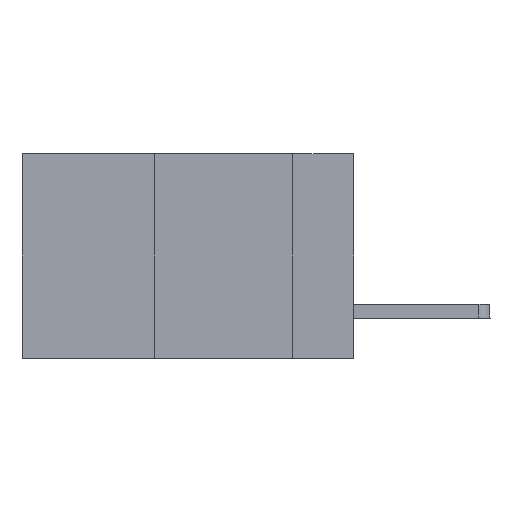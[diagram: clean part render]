
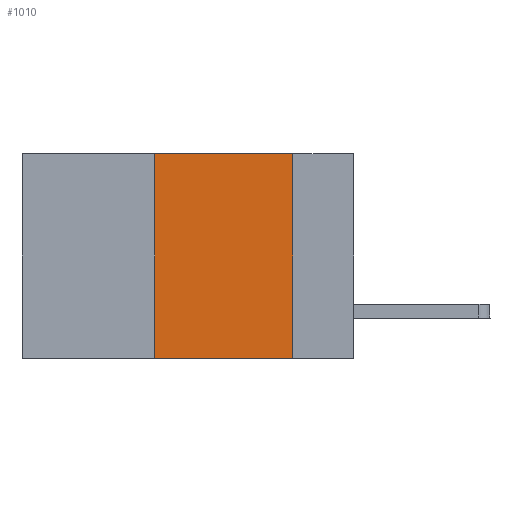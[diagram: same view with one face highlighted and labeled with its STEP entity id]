
A CAD part, left-side view. The second image highlights one B-rep face of the part: STEP entity #1010.
In plain terms, the highlighted planar face has unit normal (-1, 0, 0).
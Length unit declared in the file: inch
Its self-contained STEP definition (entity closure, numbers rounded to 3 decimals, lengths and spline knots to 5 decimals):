
#25 = VERTEX_POINT ( 'NONE', #12818 ) ;
#336 = EDGE_LOOP ( 'NONE', ( #13020, #1148, #7631, #9449 ) ) ;
#522 = CARTESIAN_POINT ( 'NONE',  ( 0., 0.11, 0. ) ) ;
#782 = CARTESIAN_POINT ( 'NONE',  ( 0., 0.11, -0.37 ) ) ;
#1010 = ADVANCED_FACE ( 'NONE', ( #8247 ), #4145, .F. ) ;
#1148 = ORIENTED_EDGE ( 'NONE', *, *, #11933, .F. ) ;
#1301 = VERTEX_POINT ( 'NONE', #7869 ) ;
#3230 = AXIS2_PLACEMENT_3D ( 'NONE', #7863, #12127, #12901 ) ;
#4145 = PLANE ( 'NONE',  #3230 ) ;
#4579 = DIRECTION ( 'NONE',  ( 0., -1., 0. ) ) ;
#4854 = VERTEX_POINT ( 'NONE', #522 ) ;
#6179 = CARTESIAN_POINT ( 'NONE',  ( 0., 0.36, 0. ) ) ;
#6302 = VECTOR ( 'NONE', #11400, 39.37008 ) ;
#6614 = VECTOR ( 'NONE', #4579, 39.37008 ) ;
#6627 = LINE ( 'NONE', #6179, #6302 ) ;
#7347 = DIRECTION ( 'NONE',  ( 0., -1., 0. ) ) ;
#7631 = ORIENTED_EDGE ( 'NONE', *, *, #13656, .F. ) ;
#7681 = VERTEX_POINT ( 'NONE', #782 ) ;
#7863 = CARTESIAN_POINT ( 'NONE',  ( 0., 0.6, 0. ) ) ;
#7869 = CARTESIAN_POINT ( 'NONE',  ( 0., 0.36, -0.37 ) ) ;
#8247 = FACE_OUTER_BOUND ( 'NONE', #336, .T. ) ;
#8863 = CARTESIAN_POINT ( 'NONE',  ( 0., 0.6, -0.37 ) ) ;
#9427 = LINE ( 'NONE', #8863, #6614 ) ;
#9449 = ORIENTED_EDGE ( 'NONE', *, *, #14064, .T. ) ;
#10041 = LINE ( 'NONE', #13588, #12757 ) ;
#10774 = DIRECTION ( 'NONE',  ( 0., 0., -1. ) ) ;
#11400 = DIRECTION ( 'NONE',  ( 0., 0., 1. ) ) ;
#11529 = EDGE_CURVE ( 'NONE', #4854, #7681, #12430, .T. ) ;
#11933 = EDGE_CURVE ( 'NONE', #25, #4854, #10041, .T. ) ;
#12114 = VECTOR ( 'NONE', #10774, 39.37008 ) ;
#12127 = DIRECTION ( 'NONE',  ( 1., 0., 0. ) ) ;
#12430 = LINE ( 'NONE', #12793, #12114 ) ;
#12757 = VECTOR ( 'NONE', #7347, 39.37008 ) ;
#12793 = CARTESIAN_POINT ( 'NONE',  ( 0., 0.11, 0. ) ) ;
#12818 = CARTESIAN_POINT ( 'NONE',  ( 0., 0.36, 0. ) ) ;
#12901 = DIRECTION ( 'NONE',  ( 0., 0., -1. ) ) ;
#13020 = ORIENTED_EDGE ( 'NONE', *, *, #11529, .F. ) ;
#13588 = CARTESIAN_POINT ( 'NONE',  ( 0., 0.6, 0. ) ) ;
#13656 = EDGE_CURVE ( 'NONE', #1301, #25, #6627, .T. ) ;
#14064 = EDGE_CURVE ( 'NONE', #1301, #7681, #9427, .T. ) ;
